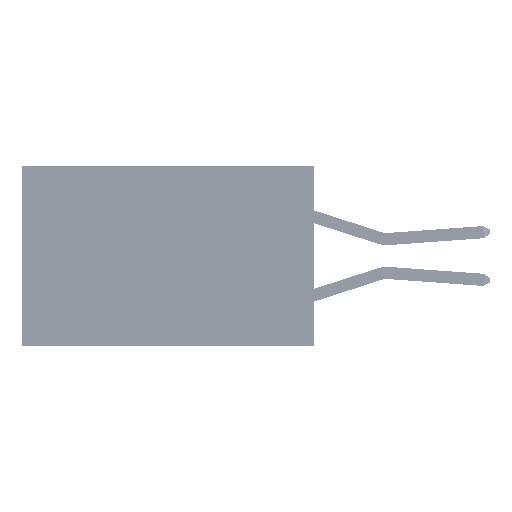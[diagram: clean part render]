
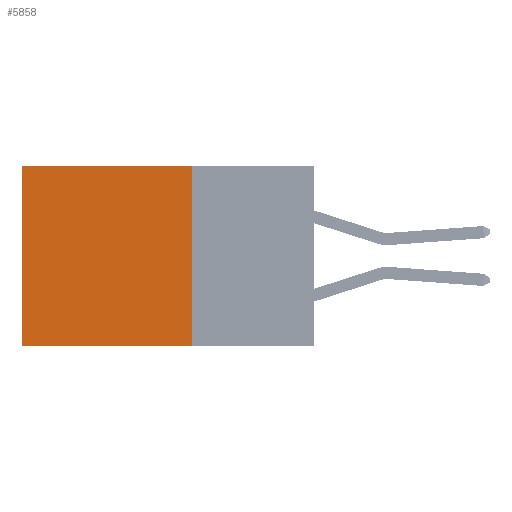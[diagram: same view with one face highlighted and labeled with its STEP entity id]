
A CAD part, left-side view. The second image highlights one B-rep face of the part: STEP entity #5858.
In plain terms, the highlighted planar face has unit normal (-1, 0, 0).
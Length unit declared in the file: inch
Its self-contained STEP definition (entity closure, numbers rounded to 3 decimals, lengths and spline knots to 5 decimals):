
#717 = VERTEX_POINT ( 'NONE', #16152 ) ;
#2554 = VERTEX_POINT ( 'NONE', #4718 ) ;
#3403 = DIRECTION ( 'NONE',  ( 0., 0., -1. ) ) ;
#4718 = CARTESIAN_POINT ( 'NONE',  ( 0.2875, 0.6, 0. ) ) ;
#4856 = CARTESIAN_POINT ( 'NONE',  ( 0.2875, 0.25, 0. ) ) ;
#5010 = DIRECTION ( 'NONE',  ( 0., 1., 0. ) ) ;
#5782 = ORIENTED_EDGE ( 'NONE', *, *, #22024, .T. ) ;
#5858 = ADVANCED_FACE ( 'NONE', ( #30545 ), #46305, .F. ) ;
#7026 = DIRECTION ( 'NONE',  ( 1., 0., 0. ) ) ;
#10913 = CARTESIAN_POINT ( 'NONE',  ( 0.2875, 0.25, 0. ) ) ;
#12621 = DIRECTION ( 'NONE',  ( 0., 0., -1. ) ) ;
#14958 = LINE ( 'NONE', #22722, #45387 ) ;
#15730 = VERTEX_POINT ( 'NONE', #28724 ) ;
#16152 = CARTESIAN_POINT ( 'NONE',  ( 0.2875, 0.25, -0.37 ) ) ;
#18285 = VECTOR ( 'NONE', #12621, 39.37008 ) ;
#18292 = EDGE_CURVE ( 'NONE', #34854, #717, #48252, .T. ) ;
#18322 = CARTESIAN_POINT ( 'NONE',  ( 0.2875, 0.25, 0. ) ) ;
#21024 = VECTOR ( 'NONE', #5010, 39.37008 ) ;
#22024 = EDGE_CURVE ( 'NONE', #2554, #15730, #14958, .T. ) ;
#22722 = CARTESIAN_POINT ( 'NONE',  ( 0.2875, 0.6, 0. ) ) ;
#24155 = CARTESIAN_POINT ( 'NONE',  ( 0.2875, 0.25, -0.37 ) ) ;
#24173 = AXIS2_PLACEMENT_3D ( 'NONE', #10913, #7026, #3403 ) ;
#25173 = CARTESIAN_POINT ( 'NONE',  ( 0.2875, 0.25, 0. ) ) ;
#25566 = ORIENTED_EDGE ( 'NONE', *, *, #45189, .T. ) ;
#28029 = EDGE_LOOP ( 'NONE', ( #5782, #28570, #46097, #25566 ) ) ;
#28050 = LINE ( 'NONE', #25173, #45145 ) ;
#28570 = ORIENTED_EDGE ( 'NONE', *, *, #29413, .F. ) ;
#28724 = CARTESIAN_POINT ( 'NONE',  ( 0.2875, 0.6, -0.37 ) ) ;
#29413 = EDGE_CURVE ( 'NONE', #717, #15730, #40410, .T. ) ;
#30545 = FACE_OUTER_BOUND ( 'NONE', #28029, .T. ) ;
#31250 = DIRECTION ( 'NONE',  ( 0., 0., -1. ) ) ;
#32913 = DIRECTION ( 'NONE',  ( 0., 1., 0. ) ) ;
#34854 = VERTEX_POINT ( 'NONE', #18322 ) ;
#40410 = LINE ( 'NONE', #24155, #21024 ) ;
#45145 = VECTOR ( 'NONE', #32913, 39.37008 ) ;
#45189 = EDGE_CURVE ( 'NONE', #34854, #2554, #28050, .T. ) ;
#45387 = VECTOR ( 'NONE', #31250, 39.37008 ) ;
#46097 = ORIENTED_EDGE ( 'NONE', *, *, #18292, .F. ) ;
#46305 = PLANE ( 'NONE',  #24173 ) ;
#48252 = LINE ( 'NONE', #4856, #18285 ) ;
